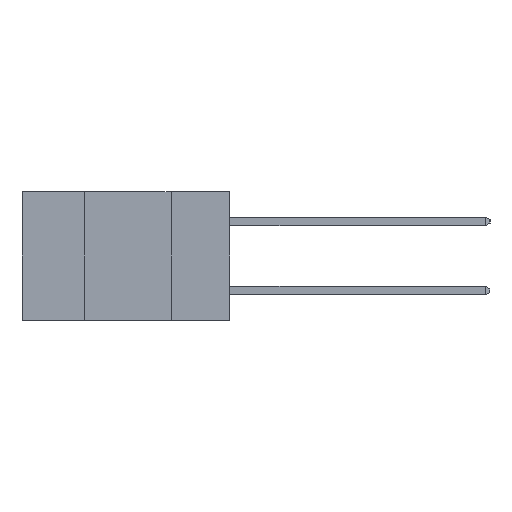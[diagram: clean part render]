
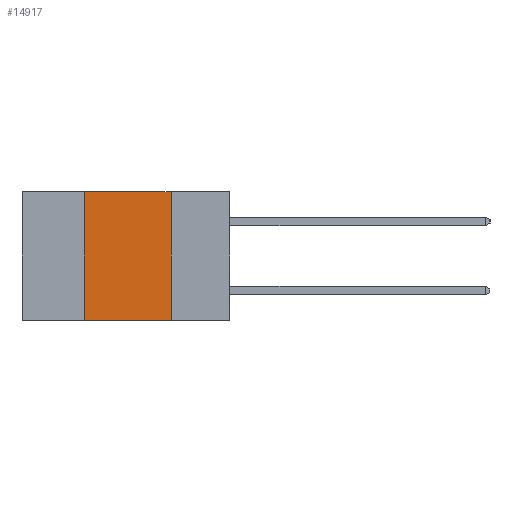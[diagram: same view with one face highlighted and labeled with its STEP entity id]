
A CAD part, left-side view. The second image highlights one B-rep face of the part: STEP entity #14917.
In plain terms, the highlighted planar face has unit normal (-1, 0, 0).
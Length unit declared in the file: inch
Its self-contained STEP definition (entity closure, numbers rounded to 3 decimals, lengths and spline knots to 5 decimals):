
#1707 = CARTESIAN_POINT ( 'NONE',  ( 0., 0.17, 0. ) ) ;
#2408 = DIRECTION ( 'NONE',  ( 1., 0., 0. ) ) ;
#2741 = CARTESIAN_POINT ( 'NONE',  ( 0., 0.42, 0. ) ) ;
#4963 = DIRECTION ( 'NONE',  ( 0., -1., 0. ) ) ;
#6052 = VERTEX_POINT ( 'NONE', #9785 ) ;
#7962 = LINE ( 'NONE', #18024, #25255 ) ;
#8352 = VERTEX_POINT ( 'NONE', #9604 ) ;
#9604 = CARTESIAN_POINT ( 'NONE',  ( 0., 0.42, -0.37 ) ) ;
#9785 = CARTESIAN_POINT ( 'NONE',  ( 0., 0.17, -0.37 ) ) ;
#9852 = EDGE_CURVE ( 'NONE', #11469, #6052, #24027, .T. ) ;
#11469 = VERTEX_POINT ( 'NONE', #17250 ) ;
#12298 = LINE ( 'NONE', #12710, #18076 ) ;
#12710 = CARTESIAN_POINT ( 'NONE',  ( 0., 0.6, 0. ) ) ;
#12786 = VECTOR ( 'NONE', #19632, 39.37008 ) ;
#13265 = CARTESIAN_POINT ( 'NONE',  ( 0., 0.6, 0. ) ) ;
#13435 = ORIENTED_EDGE ( 'NONE', *, *, #20802, .T. ) ;
#13820 = ORIENTED_EDGE ( 'NONE', *, *, #23659, .F. ) ;
#14917 = ADVANCED_FACE ( 'NONE', ( #26414 ), #26160, .F. ) ;
#14930 = AXIS2_PLACEMENT_3D ( 'NONE', #13265, #2408, #17628 ) ;
#16548 = ORIENTED_EDGE ( 'NONE', *, *, #9852, .F. ) ;
#16688 = ORIENTED_EDGE ( 'NONE', *, *, #26469, .F. ) ;
#17250 = CARTESIAN_POINT ( 'NONE',  ( 0., 0.17, 0. ) ) ;
#17437 = CARTESIAN_POINT ( 'NONE',  ( 0., 0.42, 0. ) ) ;
#17614 = VECTOR ( 'NONE', #19085, 39.37008 ) ;
#17628 = DIRECTION ( 'NONE',  ( 0., 0., -1. ) ) ;
#17877 = LINE ( 'NONE', #17437, #12786 ) ;
#18024 = CARTESIAN_POINT ( 'NONE',  ( 0., 0.6, -0.37 ) ) ;
#18076 = VECTOR ( 'NONE', #25633, 39.37008 ) ;
#19085 = DIRECTION ( 'NONE',  ( 0., 0., -1. ) ) ;
#19632 = DIRECTION ( 'NONE',  ( 0., 0., 1. ) ) ;
#20802 = EDGE_CURVE ( 'NONE', #8352, #6052, #7962, .T. ) ;
#22022 = VERTEX_POINT ( 'NONE', #2741 ) ;
#22965 = EDGE_LOOP ( 'NONE', ( #16548, #16688, #13820, #13435 ) ) ;
#23659 = EDGE_CURVE ( 'NONE', #8352, #22022, #17877, .T. ) ;
#24027 = LINE ( 'NONE', #1707, #17614 ) ;
#25255 = VECTOR ( 'NONE', #4963, 39.37008 ) ;
#25633 = DIRECTION ( 'NONE',  ( 0., -1., 0. ) ) ;
#26160 = PLANE ( 'NONE',  #14930 ) ;
#26414 = FACE_OUTER_BOUND ( 'NONE', #22965, .T. ) ;
#26469 = EDGE_CURVE ( 'NONE', #22022, #11469, #12298, .T. ) ;
